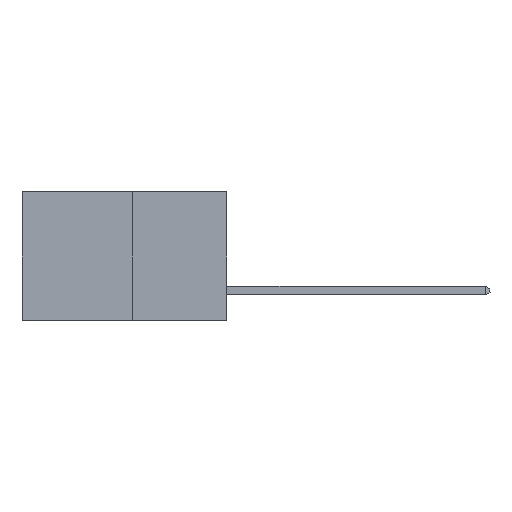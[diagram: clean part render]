
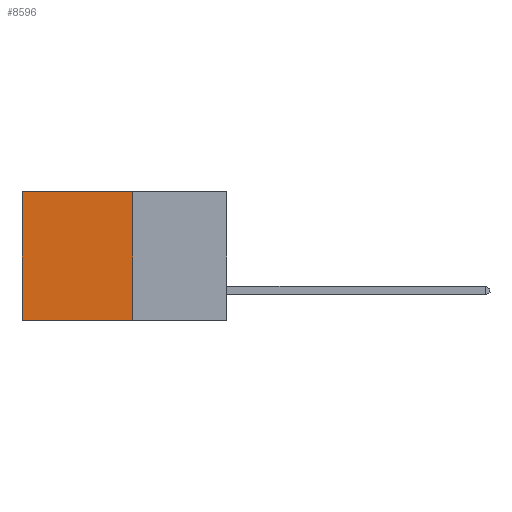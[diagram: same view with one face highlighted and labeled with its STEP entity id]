
A CAD part, left-side view. The second image highlights one B-rep face of the part: STEP entity #8596.
In plain terms, the highlighted planar face has unit normal (-1, 0, 0).
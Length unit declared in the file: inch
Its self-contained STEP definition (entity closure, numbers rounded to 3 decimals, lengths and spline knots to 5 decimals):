
#233 = CARTESIAN_POINT ( 'NONE',  ( 0.277, 0.27, 0. ) ) ;
#810 = VERTEX_POINT ( 'NONE', #1944 ) ;
#892 = LINE ( 'NONE', #12034, #6674 ) ;
#1056 = CARTESIAN_POINT ( 'NONE',  ( 0.277, 0.27, 0. ) ) ;
#1133 = DIRECTION ( 'NONE',  ( 0., 1., 0. ) ) ;
#1698 = LINE ( 'NONE', #5459, #10328 ) ;
#1944 = CARTESIAN_POINT ( 'NONE',  ( 0.277, 0.27, -0.37 ) ) ;
#3101 = FACE_OUTER_BOUND ( 'NONE', #10510, .T. ) ;
#3338 = ORIENTED_EDGE ( 'NONE', *, *, #7819, .T. ) ;
#3588 = EDGE_CURVE ( 'NONE', #810, #10600, #5495, .T. ) ;
#3657 = VERTEX_POINT ( 'NONE', #13191 ) ;
#3979 = AXIS2_PLACEMENT_3D ( 'NONE', #4483, #6746, #14143 ) ;
#4483 = CARTESIAN_POINT ( 'NONE',  ( 0.277, 0.27, -0.37 ) ) ;
#5459 = CARTESIAN_POINT ( 'NONE',  ( 0.277, 0.59, -0.37 ) ) ;
#5495 = LINE ( 'NONE', #8128, #8094 ) ;
#5645 = PLANE ( 'NONE',  #3979 ) ;
#6049 = VERTEX_POINT ( 'NONE', #1056 ) ;
#6580 = DIRECTION ( 'NONE',  ( 0., 0., -1. ) ) ;
#6674 = VECTOR ( 'NONE', #14093, 39.37008 ) ;
#6746 = DIRECTION ( 'NONE',  ( 1., 0., 0. ) ) ;
#7168 = EDGE_CURVE ( 'NONE', #6049, #3657, #11150, .T. ) ;
#7185 = ORIENTED_EDGE ( 'NONE', *, *, #3588, .F. ) ;
#7586 = ORIENTED_EDGE ( 'NONE', *, *, #13213, .F. ) ;
#7819 = EDGE_CURVE ( 'NONE', #3657, #10600, #1698, .T. ) ;
#8094 = VECTOR ( 'NONE', #1133, 39.37008 ) ;
#8128 = CARTESIAN_POINT ( 'NONE',  ( 0.277, 0.27, -0.37 ) ) ;
#8596 = ADVANCED_FACE ( 'NONE', ( #3101 ), #5645, .F. ) ;
#9405 = CARTESIAN_POINT ( 'NONE',  ( 0.277, 0.59, -0.37 ) ) ;
#10328 = VECTOR ( 'NONE', #6580, 39.37008 ) ;
#10510 = EDGE_LOOP ( 'NONE', ( #3338, #7185, #7586, #11264 ) ) ;
#10600 = VERTEX_POINT ( 'NONE', #9405 ) ;
#10838 = VECTOR ( 'NONE', #14261, 39.37008 ) ;
#11150 = LINE ( 'NONE', #233, #10838 ) ;
#11264 = ORIENTED_EDGE ( 'NONE', *, *, #7168, .T. ) ;
#12034 = CARTESIAN_POINT ( 'NONE',  ( 0.277, 0.27, -0.37 ) ) ;
#13191 = CARTESIAN_POINT ( 'NONE',  ( 0.277, 0.59, 0. ) ) ;
#13213 = EDGE_CURVE ( 'NONE', #6049, #810, #892, .T. ) ;
#14093 = DIRECTION ( 'NONE',  ( 0., 0., -1. ) ) ;
#14143 = DIRECTION ( 'NONE',  ( 0., 0., -1. ) ) ;
#14261 = DIRECTION ( 'NONE',  ( 0., 1., 0. ) ) ;
